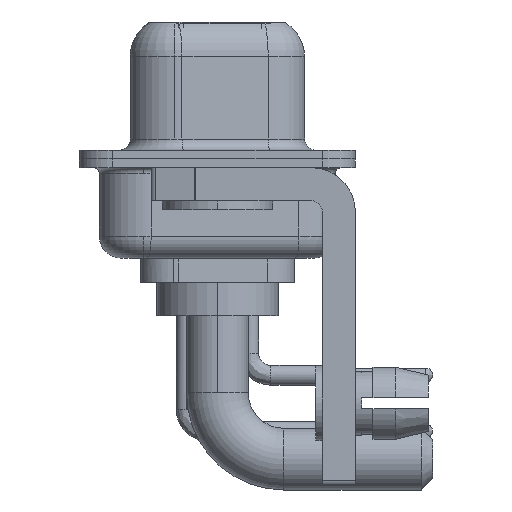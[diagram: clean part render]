
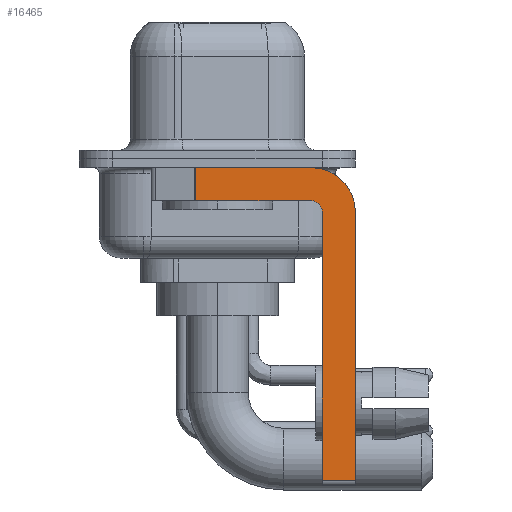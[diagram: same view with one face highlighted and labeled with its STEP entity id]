
A CAD part, left-side view. The second image highlights one B-rep face of the part: STEP entity #16465.
In plain terms, the highlighted planar face has unit normal (-1, 0, 0).
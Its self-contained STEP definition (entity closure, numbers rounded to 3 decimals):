
#17 = EDGE_LOOP ( 'NONE', ( #17888, #17749, #1294, #5533, #2048, #22222, #862, #497 ) ) ;
#497 = ORIENTED_EDGE ( 'NONE', *, *, #8410, .F. ) ;
#660 = DIRECTION ( 'NONE',  ( 0., 0., -1. ) ) ;
#862 = ORIENTED_EDGE ( 'NONE', *, *, #13773, .F. ) ;
#1024 = DIRECTION ( 'NONE',  ( 0., 0., -1. ) ) ;
#1151 = CARTESIAN_POINT ( 'NONE',  ( -2.9, -6.25, -14.55 ) ) ;
#1294 = ORIENTED_EDGE ( 'NONE', *, *, #16311, .F. ) ;
#2048 = ORIENTED_EDGE ( 'NONE', *, *, #11294, .F. ) ;
#3070 = EDGE_CURVE ( 'NONE', #7166, #16458, #4334, .T. ) ;
#4031 = CARTESIAN_POINT ( 'NONE',  ( -2.9, -4.25, -2.4 ) ) ;
#4189 = CARTESIAN_POINT ( 'NONE',  ( -2.9, -4.25, -0.4 ) ) ;
#4222 = LINE ( 'NONE', #21383, #18014 ) ;
#4334 = LINE ( 'NONE', #17454, #7926 ) ;
#4512 = EDGE_CURVE ( 'NONE', #7219, #21700, #13842, .T. ) ;
#5533 = ORIENTED_EDGE ( 'NONE', *, *, #4512, .F. ) ;
#5537 = AXIS2_PLACEMENT_3D ( 'NONE', #4031, #9820, #7855 ) ;
#5860 = LINE ( 'NONE', #22651, #19203 ) ;
#6056 = DIRECTION ( 'NONE',  ( 0., 0., -1. ) ) ;
#7166 = VERTEX_POINT ( 'NONE', #21275 ) ;
#7219 = VERTEX_POINT ( 'NONE', #8904 ) ;
#7855 = DIRECTION ( 'NONE',  ( 0., 0., 1. ) ) ;
#7926 = VECTOR ( 'NONE', #20891, 1000. ) ;
#8392 = VERTEX_POINT ( 'NONE', #19207 ) ;
#8410 = EDGE_CURVE ( 'NONE', #15787, #11747, #15918, .T. ) ;
#8438 = FACE_OUTER_BOUND ( 'NONE', #17, .T. ) ;
#8904 = CARTESIAN_POINT ( 'NONE',  ( -2.9, -4.75, -2.4 ) ) ;
#9165 = AXIS2_PLACEMENT_3D ( 'NONE', #12646, #20182, #19818 ) ;
#9633 = LINE ( 'NONE', #11254, #15551 ) ;
#9820 = DIRECTION ( 'NONE',  ( -1., 0., 0. ) ) ;
#11254 = CARTESIAN_POINT ( 'NONE',  ( -2.9, 0.978, -1.9 ) ) ;
#11294 = EDGE_CURVE ( 'NONE', #7166, #7219, #5860, .T. ) ;
#11747 = VERTEX_POINT ( 'NONE', #20183 ) ;
#11790 = DIRECTION ( 'NONE',  ( 0., 1., 0. ) ) ;
#12513 = LINE ( 'NONE', #23378, #23948 ) ;
#12646 = CARTESIAN_POINT ( 'NONE',  ( -2.9, -4.25, -2.4 ) ) ;
#13773 = EDGE_CURVE ( 'NONE', #11747, #16458, #12513, .T. ) ;
#13842 = CIRCLE ( 'NONE', #5537, 0.5 ) ;
#14690 = DIRECTION ( 'NONE',  ( 0., 0., 1. ) ) ;
#15373 = LINE ( 'NONE', #15499, #18662 ) ;
#15499 = CARTESIAN_POINT ( 'NONE',  ( -2.9, -4.25, -1.9 ) ) ;
#15551 = VECTOR ( 'NONE', #6056, 1000. ) ;
#15593 = DIRECTION ( 'NONE',  ( 0., -1., 0. ) ) ;
#15787 = VERTEX_POINT ( 'NONE', #4189 ) ;
#15918 = CIRCLE ( 'NONE', #21427, 2. ) ;
#16311 = EDGE_CURVE ( 'NONE', #21700, #22475, #15373, .T. ) ;
#16458 = VERTEX_POINT ( 'NONE', #1151 ) ;
#16465 = ADVANCED_FACE ( 'NONE', ( #8438 ), #18100, .F. ) ;
#17454 = CARTESIAN_POINT ( 'NONE',  ( -2.9, -4.25, -14.55 ) ) ;
#17487 = EDGE_CURVE ( 'NONE', #8392, #22475, #9633, .T. ) ;
#17749 = ORIENTED_EDGE ( 'NONE', *, *, #17487, .T. ) ;
#17888 = ORIENTED_EDGE ( 'NONE', *, *, #20723, .F. ) ;
#18014 = VECTOR ( 'NONE', #15593, 1000. ) ;
#18100 = PLANE ( 'NONE',  #9165 ) ;
#18662 = VECTOR ( 'NONE', #11790, 1000. ) ;
#19203 = VECTOR ( 'NONE', #14690, 1000. ) ;
#19207 = CARTESIAN_POINT ( 'NONE',  ( -2.9, 0.978, -0.4 ) ) ;
#19818 = DIRECTION ( 'NONE',  ( 0., 0., -1. ) ) ;
#20182 = DIRECTION ( 'NONE',  ( 1., 0., 0. ) ) ;
#20183 = CARTESIAN_POINT ( 'NONE',  ( -2.9, -6.25, -2.4 ) ) ;
#20723 = EDGE_CURVE ( 'NONE', #8392, #15787, #4222, .T. ) ;
#20891 = DIRECTION ( 'NONE',  ( 0., -1., 0. ) ) ;
#21034 = CARTESIAN_POINT ( 'NONE',  ( -2.9, -4.25, -2.4 ) ) ;
#21275 = CARTESIAN_POINT ( 'NONE',  ( -2.9, -4.75, -14.55 ) ) ;
#21383 = CARTESIAN_POINT ( 'NONE',  ( -2.9, 3., -0.4 ) ) ;
#21403 = DIRECTION ( 'NONE',  ( 1., 0., 0. ) ) ;
#21427 = AXIS2_PLACEMENT_3D ( 'NONE', #21034, #21403, #660 ) ;
#21679 = CARTESIAN_POINT ( 'NONE',  ( -2.9, 0.978, -1.9 ) ) ;
#21700 = VERTEX_POINT ( 'NONE', #23709 ) ;
#22222 = ORIENTED_EDGE ( 'NONE', *, *, #3070, .T. ) ;
#22475 = VERTEX_POINT ( 'NONE', #21679 ) ;
#22651 = CARTESIAN_POINT ( 'NONE',  ( -2.9, -4.75, -14.8 ) ) ;
#23378 = CARTESIAN_POINT ( 'NONE',  ( -2.9, -6.25, -2.4 ) ) ;
#23709 = CARTESIAN_POINT ( 'NONE',  ( -2.9, -4.25, -1.9 ) ) ;
#23948 = VECTOR ( 'NONE', #1024, 1000. ) ;
